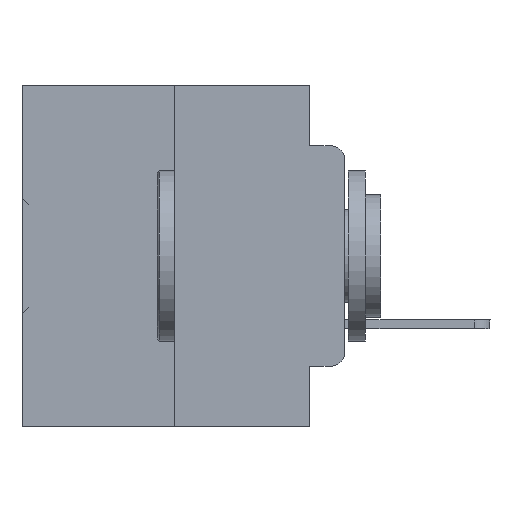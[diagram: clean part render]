
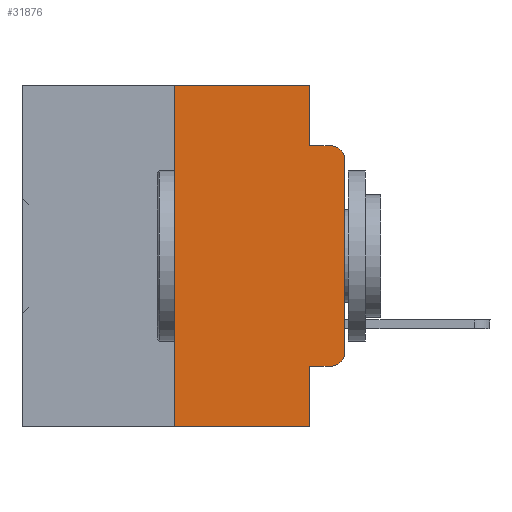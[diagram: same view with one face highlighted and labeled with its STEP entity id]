
A CAD part, left-side view. The second image highlights one B-rep face of the part: STEP entity #31876.
In plain terms, the highlighted planar face has unit normal (-1, 0, 0).
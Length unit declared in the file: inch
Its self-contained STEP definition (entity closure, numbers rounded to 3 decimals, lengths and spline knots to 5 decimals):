
#359 = EDGE_CURVE ( 'NONE', #24532, #17141, #20500, .T. ) ;
#1966 = CARTESIAN_POINT ( 'NONE',  ( 0., 0.473, 0. ) ) ;
#2256 = VECTOR ( 'NONE', #6792, 39.37008 ) ;
#2379 = VECTOR ( 'NONE', #13778, 39.37008 ) ;
#5003 = AXIS2_PLACEMENT_3D ( 'NONE', #32337, #30060, #12481 ) ;
#6109 = LINE ( 'NONE', #34054, #33633 ) ;
#6792 = DIRECTION ( 'NONE',  ( 0., -1., 0. ) ) ;
#6806 = CIRCLE ( 'NONE', #5003, 0.02 ) ;
#6973 = ORIENTED_EDGE ( 'NONE', *, *, #36741, .T. ) ;
#7929 = CARTESIAN_POINT ( 'NONE',  ( 0., 0.02, -0.1085 ) ) ;
#8068 = DIRECTION ( 'NONE',  ( 0., -1., 0. ) ) ;
#8445 = LINE ( 'NONE', #36744, #25797 ) ;
#8636 = VERTEX_POINT ( 'NONE', #28434 ) ;
#8848 = AXIS2_PLACEMENT_3D ( 'NONE', #1966, #30625, #24437 ) ;
#8925 = CARTESIAN_POINT ( 'NONE',  ( 0., 0.02, -0.0885 ) ) ;
#9955 = ORIENTED_EDGE ( 'NONE', *, *, #15609, .F. ) ;
#10114 = VECTOR ( 'NONE', #20866, 39.37008 ) ;
#10885 = VECTOR ( 'NONE', #36594, 39.37008 ) ;
#11340 = AXIS2_PLACEMENT_3D ( 'NONE', #7929, #33226, #25342 ) ;
#11802 = ORIENTED_EDGE ( 'NONE', *, *, #34729, .T. ) ;
#11841 = EDGE_CURVE ( 'NONE', #8636, #36444, #21559, .T. ) ;
#11978 = CARTESIAN_POINT ( 'NONE',  ( 0., 0.051, -0.0885 ) ) ;
#12269 = CARTESIAN_POINT ( 'NONE',  ( 0., 0., -0.3915 ) ) ;
#12481 = DIRECTION ( 'NONE',  ( 0., 0., -1. ) ) ;
#12568 = VERTEX_POINT ( 'NONE', #8925 ) ;
#13033 = FACE_OUTER_BOUND ( 'NONE', #24298, .T. ) ;
#13216 = CARTESIAN_POINT ( 'NONE',  ( 0., 0.051, 0. ) ) ;
#13778 = DIRECTION ( 'NONE',  ( 0., 0., -1. ) ) ;
#14038 = ORIENTED_EDGE ( 'NONE', *, *, #25116, .T. ) ;
#14555 = CARTESIAN_POINT ( 'NONE',  ( 0., 0., 0. ) ) ;
#14705 = ORIENTED_EDGE ( 'NONE', *, *, #18815, .F. ) ;
#15609 = EDGE_CURVE ( 'NONE', #8636, #31342, #6109, .T. ) ;
#16498 = VERTEX_POINT ( 'NONE', #11978 ) ;
#17141 = VERTEX_POINT ( 'NONE', #18808 ) ;
#17192 = EDGE_CURVE ( 'NONE', #23707, #16498, #19372, .T. ) ;
#17522 = CARTESIAN_POINT ( 'NONE',  ( 0., 0.25, 0. ) ) ;
#18005 = ORIENTED_EDGE ( 'NONE', *, *, #11841, .T. ) ;
#18808 = CARTESIAN_POINT ( 'NONE',  ( 0., 0.25, 0. ) ) ;
#18815 = EDGE_CURVE ( 'NONE', #16498, #12568, #33213, .T. ) ;
#19372 = LINE ( 'NONE', #13216, #2379 ) ;
#19650 = CARTESIAN_POINT ( 'NONE',  ( 0., 0.25, -0.5 ) ) ;
#20500 = LINE ( 'NONE', #17522, #10114 ) ;
#20748 = CARTESIAN_POINT ( 'NONE',  ( 0., 0.051, -0.5 ) ) ;
#20866 = DIRECTION ( 'NONE',  ( 0., 0., 1. ) ) ;
#21011 = LINE ( 'NONE', #34746, #34402 ) ;
#21196 = CARTESIAN_POINT ( 'NONE',  ( 0., 0.051, 0. ) ) ;
#21375 = CARTESIAN_POINT ( 'NONE',  ( 0., 0.051, -0.4115 ) ) ;
#21498 = ORIENTED_EDGE ( 'NONE', *, *, #359, .F. ) ;
#21559 = LINE ( 'NONE', #21375, #2256 ) ;
#22795 = EDGE_CURVE ( 'NONE', #36444, #34549, #6806, .T. ) ;
#23696 = EDGE_CURVE ( 'NONE', #17141, #23707, #21011, .T. ) ;
#23707 = VERTEX_POINT ( 'NONE', #21196 ) ;
#24298 = EDGE_LOOP ( 'NONE', ( #14038, #11802, #14705, #28839, #26437, #21498, #6973, #9955, #18005, #30633 ) ) ;
#24392 = CARTESIAN_POINT ( 'NONE',  ( 0., 0.051, -0.0885 ) ) ;
#24437 = DIRECTION ( 'NONE',  ( 0., 0., -1. ) ) ;
#24532 = VERTEX_POINT ( 'NONE', #19650 ) ;
#25075 = CIRCLE ( 'NONE', #11340, 0.02 ) ;
#25116 = EDGE_CURVE ( 'NONE', #34549, #26853, #28783, .T. ) ;
#25342 = DIRECTION ( 'NONE',  ( 0., 0., -1. ) ) ;
#25466 = VECTOR ( 'NONE', #34428, 39.37008 ) ;
#25591 = DIRECTION ( 'NONE',  ( 0., 0., -1. ) ) ;
#25797 = VECTOR ( 'NONE', #8068, 39.37008 ) ;
#25876 = CARTESIAN_POINT ( 'NONE',  ( 0., 0., -0.1085 ) ) ;
#26437 = ORIENTED_EDGE ( 'NONE', *, *, #23696, .F. ) ;
#26853 = VERTEX_POINT ( 'NONE', #25876 ) ;
#27443 = PLANE ( 'NONE',  #8848 ) ;
#28434 = CARTESIAN_POINT ( 'NONE',  ( 0., 0.051, -0.4115 ) ) ;
#28717 = CARTESIAN_POINT ( 'NONE',  ( 0., 0.02, -0.4115 ) ) ;
#28783 = LINE ( 'NONE', #14555, #25466 ) ;
#28839 = ORIENTED_EDGE ( 'NONE', *, *, #17192, .F. ) ;
#30060 = DIRECTION ( 'NONE',  ( -1., 0., 0. ) ) ;
#30625 = DIRECTION ( 'NONE',  ( 1., 0., 0. ) ) ;
#30633 = ORIENTED_EDGE ( 'NONE', *, *, #22795, .T. ) ;
#31342 = VERTEX_POINT ( 'NONE', #20748 ) ;
#31876 = ADVANCED_FACE ( 'NONE', ( #13033 ), #27443, .F. ) ;
#32337 = CARTESIAN_POINT ( 'NONE',  ( 0., 0.02, -0.3915 ) ) ;
#33213 = LINE ( 'NONE', #24392, #10885 ) ;
#33226 = DIRECTION ( 'NONE',  ( -1., 0., 0. ) ) ;
#33633 = VECTOR ( 'NONE', #25591, 39.37008 ) ;
#34054 = CARTESIAN_POINT ( 'NONE',  ( 0., 0.051, 0. ) ) ;
#34402 = VECTOR ( 'NONE', #35479, 39.37008 ) ;
#34428 = DIRECTION ( 'NONE',  ( 0., 0., 1. ) ) ;
#34549 = VERTEX_POINT ( 'NONE', #12269 ) ;
#34729 = EDGE_CURVE ( 'NONE', #26853, #12568, #25075, .T. ) ;
#34746 = CARTESIAN_POINT ( 'NONE',  ( 0., 0.473, 0. ) ) ;
#35479 = DIRECTION ( 'NONE',  ( 0., -1., 0. ) ) ;
#36444 = VERTEX_POINT ( 'NONE', #28717 ) ;
#36594 = DIRECTION ( 'NONE',  ( 0., -1., 0. ) ) ;
#36741 = EDGE_CURVE ( 'NONE', #24532, #31342, #8445, .T. ) ;
#36744 = CARTESIAN_POINT ( 'NONE',  ( 0., 0.473, -0.5 ) ) ;
